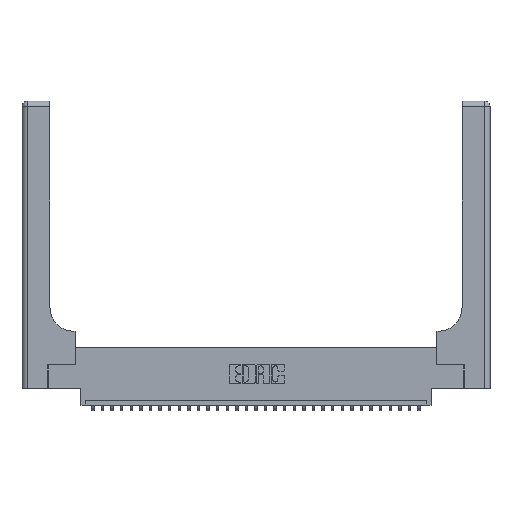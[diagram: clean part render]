
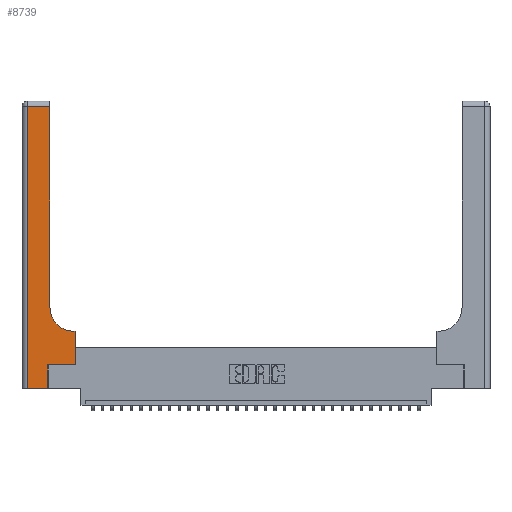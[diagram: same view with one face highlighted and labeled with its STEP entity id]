
A CAD part, top view. The second image highlights one B-rep face of the part: STEP entity #8739.
In plain terms, the highlighted planar face has unit normal (0, 0, 1).
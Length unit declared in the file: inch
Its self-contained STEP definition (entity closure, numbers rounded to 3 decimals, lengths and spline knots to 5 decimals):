
#30 = LINE ( 'NONE', #5689, #1227 ) ;
#53 = LINE ( 'NONE', #27106, #27640 ) ;
#1227 = VECTOR ( 'NONE', #28181, 39.37008 ) ;
#1289 = LINE ( 'NONE', #7768, #17853 ) ;
#3158 = EDGE_CURVE ( 'NONE', #8896, #20130, #28757, .T. ) ;
#3548 = EDGE_CURVE ( 'NONE', #10245, #13242, #5420, .T. ) ;
#4239 = EDGE_CURVE ( 'NONE', #20130, #10245, #53, .T. ) ;
#4501 = LINE ( 'NONE', #18593, #21486 ) ;
#4943 = VERTEX_POINT ( 'NONE', #10730 ) ;
#5420 = LINE ( 'NONE', #31568, #14934 ) ;
#5689 = CARTESIAN_POINT ( 'NONE',  ( 0.2915, 3., 0.37 ) ) ;
#5943 = ORIENTED_EDGE ( 'NONE', *, *, #4239, .T. ) ;
#6160 = ORIENTED_EDGE ( 'NONE', *, *, #8030, .T. ) ;
#6207 = DIRECTION ( 'NONE',  ( 1., 0., 0. ) ) ;
#6245 = CARTESIAN_POINT ( 'NONE',  ( 0.269, 0.25, 0.37 ) ) ;
#6260 = ORIENTED_EDGE ( 'NONE', *, *, #14075, .T. ) ;
#6437 = LINE ( 'NONE', #24822, #23775 ) ;
#7768 = CARTESIAN_POINT ( 'NONE',  ( 0.5585, 0.25, 0.37 ) ) ;
#8030 = EDGE_CURVE ( 'NONE', #4943, #26427, #31815, .T. ) ;
#8739 = ADVANCED_FACE ( 'NONE', ( #29790 ), #13320, .F. ) ;
#8892 = DIRECTION ( 'NONE',  ( 0., -1., 0. ) ) ;
#8896 = VERTEX_POINT ( 'NONE', #10908 ) ;
#9433 = DIRECTION ( 'NONE',  ( 0., 1., 0. ) ) ;
#10245 = VERTEX_POINT ( 'NONE', #6245 ) ;
#10730 = CARTESIAN_POINT ( 'NONE',  ( 0.2915, 2.94, 0.37 ) ) ;
#10908 = CARTESIAN_POINT ( 'NONE',  ( 0.06, 0., 0.37 ) ) ;
#10969 = CARTESIAN_POINT ( 'NONE',  ( 0.5415, 0.6, 0.37 ) ) ;
#13242 = VERTEX_POINT ( 'NONE', #25691 ) ;
#13320 = PLANE ( 'NONE',  #22294 ) ;
#13402 = ORIENTED_EDGE ( 'NONE', *, *, #3158, .T. ) ;
#14075 = EDGE_CURVE ( 'NONE', #17238, #17371, #6437, .T. ) ;
#14858 = VECTOR ( 'NONE', #25524, 39.37008 ) ;
#14934 = VECTOR ( 'NONE', #6207, 39.37008 ) ;
#15504 = CARTESIAN_POINT ( 'NONE',  ( 0.06, 2.94, 0.37 ) ) ;
#17238 = VERTEX_POINT ( 'NONE', #30204 ) ;
#17371 = VERTEX_POINT ( 'NONE', #10969 ) ;
#17596 = EDGE_CURVE ( 'NONE', #17371, #22858, #21939, .T. ) ;
#17853 = VECTOR ( 'NONE', #25550, 39.37008 ) ;
#18012 = AXIS2_PLACEMENT_3D ( 'NONE', #23760, #19358, #29282 ) ;
#18357 = DIRECTION ( 'NONE',  ( 0., 0., -1. ) ) ;
#18593 = CARTESIAN_POINT ( 'NONE',  ( 0.06, 3., 0.37 ) ) ;
#18819 = ORIENTED_EDGE ( 'NONE', *, *, #3548, .T. ) ;
#19188 = ORIENTED_EDGE ( 'NONE', *, *, #28442, .T. ) ;
#19358 = DIRECTION ( 'NONE',  ( 0., 0., -1. ) ) ;
#20119 = EDGE_CURVE ( 'NONE', #22858, #4943, #30, .T. ) ;
#20130 = VERTEX_POINT ( 'NONE', #20667 ) ;
#20667 = CARTESIAN_POINT ( 'NONE',  ( 0.269, 0., 0.37 ) ) ;
#21486 = VECTOR ( 'NONE', #8892, 39.37008 ) ;
#21939 = CIRCLE ( 'NONE', #18012, 0.25 ) ;
#22294 = AXIS2_PLACEMENT_3D ( 'NONE', #30928, #18357, #31053 ) ;
#22423 = EDGE_LOOP ( 'NONE', ( #29604, #6160, #30213, #13402, #5943, #18819, #19188, #6260, #29584 ) ) ;
#22858 = VERTEX_POINT ( 'NONE', #25359 ) ;
#23760 = CARTESIAN_POINT ( 'NONE',  ( 0.5415, 0.85, 0.37 ) ) ;
#23775 = VECTOR ( 'NONE', #27356, 39.37008 ) ;
#24822 = CARTESIAN_POINT ( 'NONE',  ( 0.2915, 0.6, 0.37 ) ) ;
#25359 = CARTESIAN_POINT ( 'NONE',  ( 0.2915, 0.85, 0.37 ) ) ;
#25511 = DIRECTION ( 'NONE',  ( 1., 0., 0. ) ) ;
#25524 = DIRECTION ( 'NONE',  ( -1., 0., 0. ) ) ;
#25550 = DIRECTION ( 'NONE',  ( 0., 1., 0. ) ) ;
#25691 = CARTESIAN_POINT ( 'NONE',  ( 0.5585, 0.25, 0.37 ) ) ;
#26427 = VERTEX_POINT ( 'NONE', #15504 ) ;
#26511 = EDGE_CURVE ( 'NONE', #26427, #8896, #4501, .T. ) ;
#26812 = VECTOR ( 'NONE', #25511, 39.37008 ) ;
#27106 = CARTESIAN_POINT ( 'NONE',  ( 0.269, 0., 0.37 ) ) ;
#27356 = DIRECTION ( 'NONE',  ( -1., 0., 0. ) ) ;
#27640 = VECTOR ( 'NONE', #9433, 39.37008 ) ;
#28181 = DIRECTION ( 'NONE',  ( 0., 1., 0. ) ) ;
#28442 = EDGE_CURVE ( 'NONE', #13242, #17238, #1289, .T. ) ;
#28757 = LINE ( 'NONE', #30049, #26812 ) ;
#29282 = DIRECTION ( 'NONE',  ( 1., 0., 0. ) ) ;
#29584 = ORIENTED_EDGE ( 'NONE', *, *, #17596, .T. ) ;
#29604 = ORIENTED_EDGE ( 'NONE', *, *, #20119, .T. ) ;
#29790 = FACE_OUTER_BOUND ( 'NONE', #22423, .T. ) ;
#30049 = CARTESIAN_POINT ( 'NONE',  ( 0., 0., 0.37 ) ) ;
#30204 = CARTESIAN_POINT ( 'NONE',  ( 0.5585, 0.6, 0.37 ) ) ;
#30213 = ORIENTED_EDGE ( 'NONE', *, *, #26511, .T. ) ;
#30928 = CARTESIAN_POINT ( 'NONE',  ( 0., 3., 0.37 ) ) ;
#31053 = DIRECTION ( 'NONE',  ( -1., 0., 0. ) ) ;
#31568 = CARTESIAN_POINT ( 'NONE',  ( 0.269, 0.25, 0.37 ) ) ;
#31815 = LINE ( 'NONE', #32060, #14858 ) ;
#32060 = CARTESIAN_POINT ( 'NONE',  ( 0., 2.94, 0.37 ) ) ;
